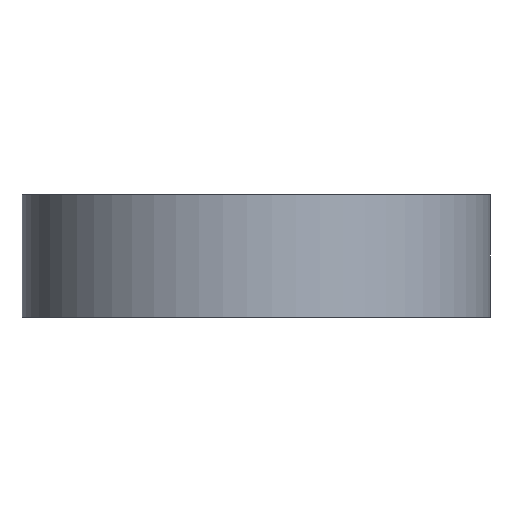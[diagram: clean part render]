
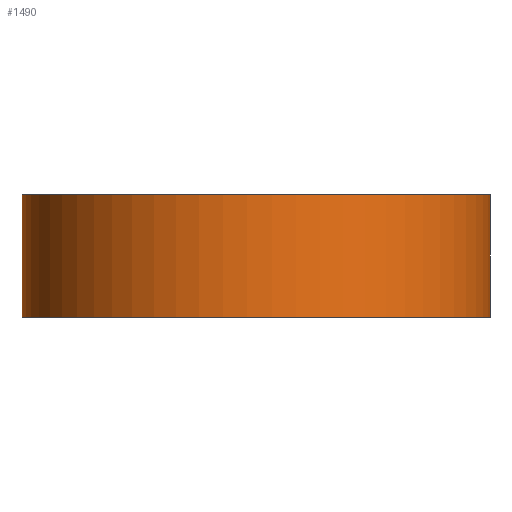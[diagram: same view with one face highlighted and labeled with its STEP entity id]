
A CAD part, front view. The second image highlights one B-rep face of the part: STEP entity #1490.
In plain terms, the highlighted free-form (B-spline) face has degree [5, 1] with [25, 2] control points.
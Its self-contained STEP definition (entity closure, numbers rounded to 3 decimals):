
#15=(
BOUNDED_SURFACE()
B_SPLINE_SURFACE(5,1,((#3183,#3184),(#3185,#3186),(#3187,#3188),(#3189,
#3190),(#3191,#3192),(#3193,#3194),(#3195,#3196),(#3197,#3198),(#3199,#3200),
(#3201,#3202),(#3203,#3204),(#3205,#3206),(#3207,#3208),(#3209,#3210),(#3211,
#3212),(#3213,#3214),(#3215,#3216),(#3217,#3218),(#3219,#3220),(#3221,#3222),
(#3223,#3224),(#3225,#3226),(#3227,#3228),(#3229,#3230),(#3231,#3232)),
 .UNSPECIFIED.,.T.,.F.,.F.)
B_SPLINE_SURFACE_WITH_KNOTS((6,1,1,1,1,1,1,1,1,1,1,1,1,1,1,1,1,1,1,1,6),
(2,2),(0.,0.05,0.1,0.15,0.2,0.25,0.3,0.35,0.4,0.45,0.5,0.55,0.6,0.65,0.7,
0.75,0.8,0.85,0.9,0.95,1.),(0.,1.),.UNSPECIFIED.)
GEOMETRIC_REPRESENTATION_ITEM()
RATIONAL_B_SPLINE_SURFACE(((1.,1.),(1.,1.),(1.,1.),(1.,1.),(1.,1.),(1.,
1.),(1.,1.),(1.,1.),(1.,1.),(1.,1.),(1.,1.),(1.,1.),(1.,1.),(1.,1.),(1.,
1.),(1.,1.),(1.,1.),(1.,1.),(1.,1.),(1.,1.),(1.,1.),(1.,1.),(1.,1.),(1.,
1.),(1.,1.)))
REPRESENTATION_ITEM('')
SURFACE()
);
#34=(
BOUNDED_CURVE()
B_SPLINE_CURVE(5,(#3121,#3122,#3123,#3124,#3125,#3126,#3127,#3128,#3129,
#3130,#3131,#3132,#3133,#3134,#3135,#3136,#3137,#3138,#3139,#3140,#3141,
#3142,#3143,#3144,#3145),.UNSPECIFIED.,.T.,.F.)
B_SPLINE_CURVE_WITH_KNOTS((6,1,1,1,1,1,1,1,1,1,1,1,1,1,1,1,1,1,1,1,6),(0.,
0.05,0.1,0.15,0.2,0.25,0.3,0.35,0.4,0.45,0.5,0.55,0.6,0.65,0.7,0.75,0.8,
0.85,0.9,0.95,1.),.UNSPECIFIED.)
CURVE()
GEOMETRIC_REPRESENTATION_ITEM()
RATIONAL_B_SPLINE_CURVE((1.,1.,1.,1.,1.,1.,1.,1.,1.,1.,1.,1.,1.,1.,1.,1.,
1.,1.,1.,1.,1.,1.,1.,1.,1.))
REPRESENTATION_ITEM('')
);
#35=(
BOUNDED_CURVE()
B_SPLINE_CURVE(5,(#3234,#3235,#3236,#3237,#3238,#3239,#3240,#3241,#3242,
#3243,#3244,#3245,#3246,#3247,#3248,#3249,#3250,#3251,#3252,#3253,#3254,
#3255,#3256,#3257,#3258),.UNSPECIFIED.,.T.,.F.)
B_SPLINE_CURVE_WITH_KNOTS((6,1,1,1,1,1,1,1,1,1,1,1,1,1,1,1,1,1,1,1,6),(0.,
0.05,0.1,0.15,0.2,0.25,0.3,0.35,0.4,0.45,0.5,0.55,0.6,0.65,0.7,0.75,0.8,
0.85,0.9,0.95,1.),.UNSPECIFIED.)
CURVE()
GEOMETRIC_REPRESENTATION_ITEM()
RATIONAL_B_SPLINE_CURVE((1.,1.,1.,1.,1.,1.,1.,1.,1.,1.,1.,1.,1.,1.,1.,1.,
1.,1.,1.,1.,1.,1.,1.,1.,1.))
REPRESENTATION_ITEM('')
);
#143=FACE_OUTER_BOUND('',#234,.T.);
#234=EDGE_LOOP('',(#1333,#1334,#1335,#1336));
#329=LINE('',#3259,#417);
#417=VECTOR('',#1688,10.);
#672=VERTEX_POINT('',#3120);
#685=VERTEX_POINT('',#3233);
#887=EDGE_CURVE('',#672,#672,#34,.T.);
#906=EDGE_CURVE('',#685,#685,#35,.T.);
#907=EDGE_CURVE('',#685,#672,#329,.T.);
#1333=ORIENTED_EDGE('',*,*,#906,.T.);
#1334=ORIENTED_EDGE('',*,*,#907,.T.);
#1335=ORIENTED_EDGE('',*,*,#887,.F.);
#1336=ORIENTED_EDGE('',*,*,#907,.F.);
#1490=ADVANCED_FACE('',(#143),#15,.T.);
#1688=DIRECTION('',(0.,0.,1.));
#3120=CARTESIAN_POINT('',(34.891,38.999,48.8));
#3121=CARTESIAN_POINT('Ctrl Pts',(34.891,38.999,48.8));
#3122=CARTESIAN_POINT('Ctrl Pts',(33.697,38.996,48.8));
#3123=CARTESIAN_POINT('Ctrl Pts',(31.309,38.801,48.8));
#3124=CARTESIAN_POINT('Ctrl Pts',(27.791,37.938,48.8));
#3125=CARTESIAN_POINT('Ctrl Pts',(23.451,35.693,48.8));
#3126=CARTESIAN_POINT('Ctrl Pts',(19.131,31.359,48.8));
#3127=CARTESIAN_POINT('Ctrl Pts',(16.346,25.925,48.8));
#3128=CARTESIAN_POINT('Ctrl Pts',(15.389,19.912,48.8));
#3129=CARTESIAN_POINT('Ctrl Pts',(16.375,13.885,48.8));
#3130=CARTESIAN_POINT('Ctrl Pts',(19.186,8.42,48.8));
#3131=CARTESIAN_POINT('Ctrl Pts',(23.524,4.05,48.8));
#3132=CARTESIAN_POINT('Ctrl Pts',(28.959,1.224,48.8));
#3133=CARTESIAN_POINT('Ctrl Pts',(34.972,0.251,48.8));
#3134=CARTESIAN_POINT('Ctrl Pts',(40.995,1.253,48.8));
#3135=CARTESIAN_POINT('Ctrl Pts',(46.456,4.105,48.8));
#3136=CARTESIAN_POINT('Ctrl Pts',(50.821,8.493,48.8));
#3137=CARTESIAN_POINT('Ctrl Pts',(53.645,13.969,48.8));
#3138=CARTESIAN_POINT('Ctrl Pts',(54.618,19.998,48.8));
#3139=CARTESIAN_POINT('Ctrl Pts',(53.62,26.005,48.8));
#3140=CARTESIAN_POINT('Ctrl Pts',(50.773,31.425,48.8));
#3141=CARTESIAN_POINT('Ctrl Pts',(46.389,35.741,48.8));
#3142=CARTESIAN_POINT('Ctrl Pts',(42.01,37.967,48.8));
#3143=CARTESIAN_POINT('Ctrl Pts',(38.476,38.816,48.8));
#3144=CARTESIAN_POINT('Ctrl Pts',(36.086,39.001,48.8));
#3145=CARTESIAN_POINT('Ctrl Pts',(34.891,38.999,48.8));
#3183=CARTESIAN_POINT('Ctrl Pts',(34.891,38.999,38.8));
#3184=CARTESIAN_POINT('Ctrl Pts',(34.891,38.999,48.8));
#3185=CARTESIAN_POINT('Ctrl Pts',(33.697,38.996,38.8));
#3186=CARTESIAN_POINT('Ctrl Pts',(33.697,38.996,48.8));
#3187=CARTESIAN_POINT('Ctrl Pts',(31.309,38.801,38.8));
#3188=CARTESIAN_POINT('Ctrl Pts',(31.309,38.801,48.8));
#3189=CARTESIAN_POINT('Ctrl Pts',(27.791,37.938,38.8));
#3190=CARTESIAN_POINT('Ctrl Pts',(27.791,37.938,48.8));
#3191=CARTESIAN_POINT('Ctrl Pts',(23.451,35.693,38.8));
#3192=CARTESIAN_POINT('Ctrl Pts',(23.451,35.693,48.8));
#3193=CARTESIAN_POINT('Ctrl Pts',(19.131,31.359,38.8));
#3194=CARTESIAN_POINT('Ctrl Pts',(19.131,31.359,48.8));
#3195=CARTESIAN_POINT('Ctrl Pts',(16.346,25.925,38.8));
#3196=CARTESIAN_POINT('Ctrl Pts',(16.346,25.925,48.8));
#3197=CARTESIAN_POINT('Ctrl Pts',(15.389,19.912,38.8));
#3198=CARTESIAN_POINT('Ctrl Pts',(15.389,19.912,48.8));
#3199=CARTESIAN_POINT('Ctrl Pts',(16.375,13.885,38.8));
#3200=CARTESIAN_POINT('Ctrl Pts',(16.375,13.885,48.8));
#3201=CARTESIAN_POINT('Ctrl Pts',(19.186,8.42,38.8));
#3202=CARTESIAN_POINT('Ctrl Pts',(19.186,8.42,48.8));
#3203=CARTESIAN_POINT('Ctrl Pts',(23.524,4.05,38.8));
#3204=CARTESIAN_POINT('Ctrl Pts',(23.524,4.05,48.8));
#3205=CARTESIAN_POINT('Ctrl Pts',(28.959,1.224,38.8));
#3206=CARTESIAN_POINT('Ctrl Pts',(28.959,1.224,48.8));
#3207=CARTESIAN_POINT('Ctrl Pts',(34.972,0.251,38.8));
#3208=CARTESIAN_POINT('Ctrl Pts',(34.972,0.251,48.8));
#3209=CARTESIAN_POINT('Ctrl Pts',(40.995,1.253,38.8));
#3210=CARTESIAN_POINT('Ctrl Pts',(40.995,1.253,48.8));
#3211=CARTESIAN_POINT('Ctrl Pts',(46.456,4.105,38.8));
#3212=CARTESIAN_POINT('Ctrl Pts',(46.456,4.105,48.8));
#3213=CARTESIAN_POINT('Ctrl Pts',(50.821,8.493,38.8));
#3214=CARTESIAN_POINT('Ctrl Pts',(50.821,8.493,48.8));
#3215=CARTESIAN_POINT('Ctrl Pts',(53.645,13.969,38.8));
#3216=CARTESIAN_POINT('Ctrl Pts',(53.645,13.969,48.8));
#3217=CARTESIAN_POINT('Ctrl Pts',(54.618,19.998,38.8));
#3218=CARTESIAN_POINT('Ctrl Pts',(54.618,19.998,48.8));
#3219=CARTESIAN_POINT('Ctrl Pts',(53.62,26.005,38.8));
#3220=CARTESIAN_POINT('Ctrl Pts',(53.62,26.005,48.8));
#3221=CARTESIAN_POINT('Ctrl Pts',(50.773,31.425,38.8));
#3222=CARTESIAN_POINT('Ctrl Pts',(50.773,31.425,48.8));
#3223=CARTESIAN_POINT('Ctrl Pts',(46.389,35.741,38.8));
#3224=CARTESIAN_POINT('Ctrl Pts',(46.389,35.741,48.8));
#3225=CARTESIAN_POINT('Ctrl Pts',(42.01,37.967,38.8));
#3226=CARTESIAN_POINT('Ctrl Pts',(42.01,37.967,48.8));
#3227=CARTESIAN_POINT('Ctrl Pts',(38.476,38.816,38.8));
#3228=CARTESIAN_POINT('Ctrl Pts',(38.476,38.816,48.8));
#3229=CARTESIAN_POINT('Ctrl Pts',(36.086,39.001,38.8));
#3230=CARTESIAN_POINT('Ctrl Pts',(36.086,39.001,48.8));
#3231=CARTESIAN_POINT('Ctrl Pts',(34.891,38.999,38.8));
#3232=CARTESIAN_POINT('Ctrl Pts',(34.891,38.999,48.8));
#3233=CARTESIAN_POINT('',(34.891,38.999,38.8));
#3234=CARTESIAN_POINT('Ctrl Pts',(34.891,38.999,38.8));
#3235=CARTESIAN_POINT('Ctrl Pts',(33.697,38.996,38.8));
#3236=CARTESIAN_POINT('Ctrl Pts',(31.309,38.801,38.8));
#3237=CARTESIAN_POINT('Ctrl Pts',(27.791,37.938,38.8));
#3238=CARTESIAN_POINT('Ctrl Pts',(23.451,35.693,38.8));
#3239=CARTESIAN_POINT('Ctrl Pts',(19.131,31.359,38.8));
#3240=CARTESIAN_POINT('Ctrl Pts',(16.346,25.925,38.8));
#3241=CARTESIAN_POINT('Ctrl Pts',(15.389,19.912,38.8));
#3242=CARTESIAN_POINT('Ctrl Pts',(16.375,13.885,38.8));
#3243=CARTESIAN_POINT('Ctrl Pts',(19.186,8.42,38.8));
#3244=CARTESIAN_POINT('Ctrl Pts',(23.524,4.05,38.8));
#3245=CARTESIAN_POINT('Ctrl Pts',(28.959,1.224,38.8));
#3246=CARTESIAN_POINT('Ctrl Pts',(34.972,0.251,38.8));
#3247=CARTESIAN_POINT('Ctrl Pts',(40.995,1.253,38.8));
#3248=CARTESIAN_POINT('Ctrl Pts',(46.456,4.105,38.8));
#3249=CARTESIAN_POINT('Ctrl Pts',(50.821,8.493,38.8));
#3250=CARTESIAN_POINT('Ctrl Pts',(53.645,13.969,38.8));
#3251=CARTESIAN_POINT('Ctrl Pts',(54.618,19.998,38.8));
#3252=CARTESIAN_POINT('Ctrl Pts',(53.62,26.005,38.8));
#3253=CARTESIAN_POINT('Ctrl Pts',(50.773,31.425,38.8));
#3254=CARTESIAN_POINT('Ctrl Pts',(46.389,35.741,38.8));
#3255=CARTESIAN_POINT('Ctrl Pts',(42.01,37.967,38.8));
#3256=CARTESIAN_POINT('Ctrl Pts',(38.476,38.816,38.8));
#3257=CARTESIAN_POINT('Ctrl Pts',(36.086,39.001,38.8));
#3258=CARTESIAN_POINT('Ctrl Pts',(34.891,38.999,38.8));
#3259=CARTESIAN_POINT('',(34.891,38.999,38.8));
